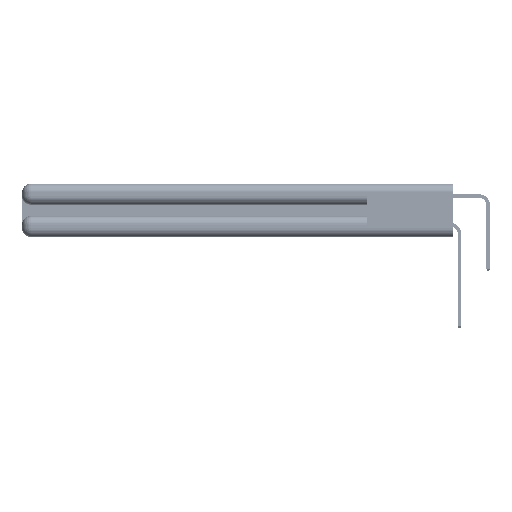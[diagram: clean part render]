
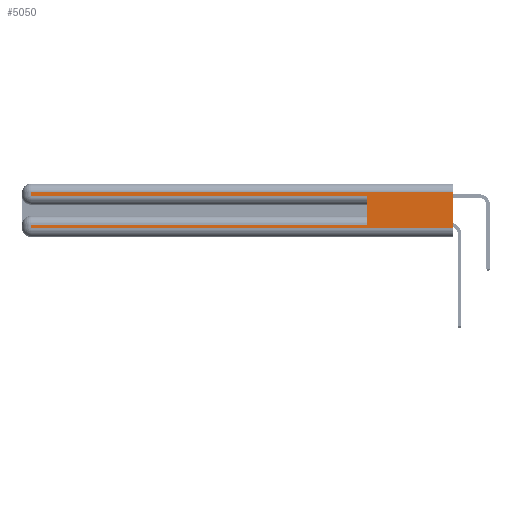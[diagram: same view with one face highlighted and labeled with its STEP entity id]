
A CAD part, left-side view. The second image highlights one B-rep face of the part: STEP entity #5050.
In plain terms, the highlighted planar face has unit normal (-1, 0, 0).
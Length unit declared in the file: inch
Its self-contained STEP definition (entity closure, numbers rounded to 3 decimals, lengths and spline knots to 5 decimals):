
#1429 = ORIENTED_EDGE ( 'NONE', *, *, #10820, .T. ) ;
#4990 = DIRECTION ( 'NONE',  ( 0., -1., 0. ) ) ;
#5050 = ADVANCED_FACE ( 'NONE', ( #23955 ), #57647, .F. ) ;
#5579 = EDGE_CURVE ( 'NONE', #8633, #51936, #42118, .T. ) ;
#6534 = VERTEX_POINT ( 'NONE', #53644 ) ;
#7465 = EDGE_CURVE ( 'NONE', #23688, #8633, #10498, .T. ) ;
#7726 = CARTESIAN_POINT ( 'NONE',  ( 0., 2.94, 0.285 ) ) ;
#8058 = CARTESIAN_POINT ( 'NONE',  ( 0., 0.6, 0.285 ) ) ;
#8310 = CARTESIAN_POINT ( 'NONE',  ( 0., 0., 0.085 ) ) ;
#8524 = DIRECTION ( 'NONE',  ( 0., 0., -1. ) ) ;
#8633 = VERTEX_POINT ( 'NONE', #7726 ) ;
#8765 = CARTESIAN_POINT ( 'NONE',  ( 0., 0., 0.31 ) ) ;
#10498 = LINE ( 'NONE', #38477, #46273 ) ;
#10820 = EDGE_CURVE ( 'NONE', #10832, #6534, #28350, .T. ) ;
#10832 = VERTEX_POINT ( 'NONE', #32056 ) ;
#11834 = ORIENTED_EDGE ( 'NONE', *, *, #7465, .T. ) ;
#12626 = VECTOR ( 'NONE', #38372, 39.37008 ) ;
#15745 = EDGE_CURVE ( 'NONE', #34256, #44570, #54502, .T. ) ;
#16089 = CARTESIAN_POINT ( 'NONE',  ( 0., 2.94, 0.085 ) ) ;
#16753 = ORIENTED_EDGE ( 'NONE', *, *, #29710, .F. ) ;
#17690 = CARTESIAN_POINT ( 'NONE',  ( 0., 2.94, 0.37 ) ) ;
#20279 = CARTESIAN_POINT ( 'NONE',  ( 0., 0.6, 0.145 ) ) ;
#20365 = ORIENTED_EDGE ( 'NONE', *, *, #15745, .T. ) ;
#20650 = DIRECTION ( 'NONE',  ( 0., -1., 0. ) ) ;
#22826 = CARTESIAN_POINT ( 'NONE',  ( 0., 0., 0.06 ) ) ;
#23688 = VERTEX_POINT ( 'NONE', #52500 ) ;
#23955 = FACE_OUTER_BOUND ( 'NONE', #52068, .T. ) ;
#24520 = LINE ( 'NONE', #47195, #12626 ) ;
#24724 = CARTESIAN_POINT ( 'NONE',  ( 0., 0.6, 0.085 ) ) ;
#25517 = EDGE_CURVE ( 'NONE', #33231, #23688, #24520, .T. ) ;
#26011 = ORIENTED_EDGE ( 'NONE', *, *, #31865, .T. ) ;
#28097 = LINE ( 'NONE', #17690, #54695 ) ;
#28350 = LINE ( 'NONE', #22826, #50779 ) ;
#28654 = ORIENTED_EDGE ( 'NONE', *, *, #25517, .T. ) ;
#29710 = EDGE_CURVE ( 'NONE', #33231, #6534, #31063, .T. ) ;
#30883 = CARTESIAN_POINT ( 'NONE',  ( 0., 0., 0.37 ) ) ;
#31063 = LINE ( 'NONE', #56630, #41557 ) ;
#31083 = VECTOR ( 'NONE', #42608, 39.37008 ) ;
#31865 = EDGE_CURVE ( 'NONE', #44570, #10832, #28097, .T. ) ;
#32056 = CARTESIAN_POINT ( 'NONE',  ( 0., 2.94, 0.06 ) ) ;
#33231 = VERTEX_POINT ( 'NONE', #8765 ) ;
#33590 = ORIENTED_EDGE ( 'NONE', *, *, #5579, .T. ) ;
#34256 = VERTEX_POINT ( 'NONE', #24724 ) ;
#35386 = DIRECTION ( 'NONE',  ( 1., 0., 0. ) ) ;
#36743 = EDGE_CURVE ( 'NONE', #34256, #51936, #42981, .T. ) ;
#38372 = DIRECTION ( 'NONE',  ( 0., 1., 0. ) ) ;
#38477 = CARTESIAN_POINT ( 'NONE',  ( 0., 2.94, 0.37 ) ) ;
#39321 = VECTOR ( 'NONE', #20650, 39.37008 ) ;
#41557 = VECTOR ( 'NONE', #43349, 39.37008 ) ;
#42118 = LINE ( 'NONE', #43158, #39321 ) ;
#42608 = DIRECTION ( 'NONE',  ( 0., 0., 1. ) ) ;
#42981 = LINE ( 'NONE', #20279, #31083 ) ;
#43158 = CARTESIAN_POINT ( 'NONE',  ( 0., 0., 0.285 ) ) ;
#43349 = DIRECTION ( 'NONE',  ( 0., 0., -1. ) ) ;
#44187 = DIRECTION ( 'NONE',  ( 0., 1., 0. ) ) ;
#44570 = VERTEX_POINT ( 'NONE', #16089 ) ;
#46273 = VECTOR ( 'NONE', #47302, 39.37008 ) ;
#46976 = ORIENTED_EDGE ( 'NONE', *, *, #36743, .F. ) ;
#47195 = CARTESIAN_POINT ( 'NONE',  ( 0., 0., 0.31 ) ) ;
#47293 = AXIS2_PLACEMENT_3D ( 'NONE', #30883, #35386, #8524 ) ;
#47302 = DIRECTION ( 'NONE',  ( 0., 0., -1. ) ) ;
#50779 = VECTOR ( 'NONE', #4990, 39.37008 ) ;
#51936 = VERTEX_POINT ( 'NONE', #8058 ) ;
#52068 = EDGE_LOOP ( 'NONE', ( #16753, #28654, #11834, #33590, #46976, #20365, #26011, #1429 ) ) ;
#52500 = CARTESIAN_POINT ( 'NONE',  ( 0., 2.94, 0.31 ) ) ;
#53138 = VECTOR ( 'NONE', #44187, 39.37008 ) ;
#53644 = CARTESIAN_POINT ( 'NONE',  ( 0., 0., 0.06 ) ) ;
#53708 = DIRECTION ( 'NONE',  ( 0., 0., -1. ) ) ;
#54502 = LINE ( 'NONE', #8310, #53138 ) ;
#54695 = VECTOR ( 'NONE', #53708, 39.37008 ) ;
#56630 = CARTESIAN_POINT ( 'NONE',  ( 0., 0., 0.37 ) ) ;
#57647 = PLANE ( 'NONE',  #47293 ) ;
